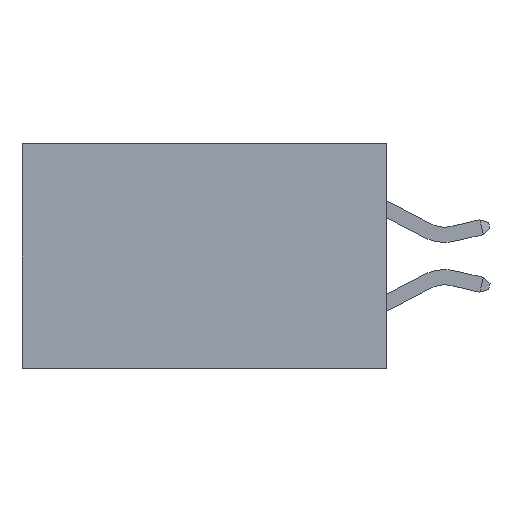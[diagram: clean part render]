
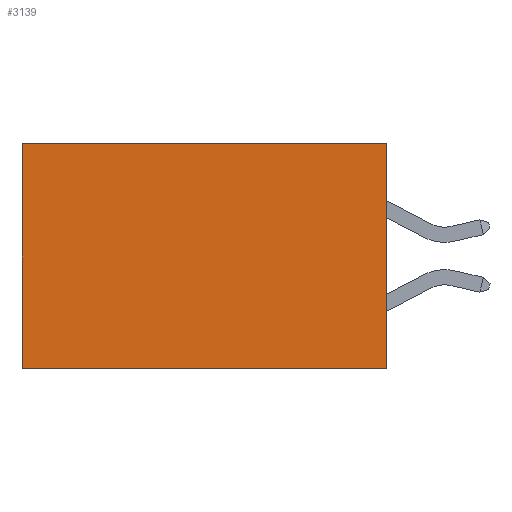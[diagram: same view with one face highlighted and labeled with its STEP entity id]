
A CAD part, left-side view. The second image highlights one B-rep face of the part: STEP entity #3139.
In plain terms, the highlighted planar face has unit normal (-1, 0, 0).
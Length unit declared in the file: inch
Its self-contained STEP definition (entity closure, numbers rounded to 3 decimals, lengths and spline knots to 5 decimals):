
#205 = VECTOR ( 'NONE', #7128, 39.37008 ) ;
#411 = LINE ( 'NONE', #13091, #9566 ) ;
#549 = VERTEX_POINT ( 'NONE', #5265 ) ;
#751 = LINE ( 'NONE', #3924, #11899 ) ;
#807 = DIRECTION ( 'NONE',  ( 0., 0., -1. ) ) ;
#1482 = VERTEX_POINT ( 'NONE', #13178 ) ;
#1638 = DIRECTION ( 'NONE',  ( 0., 1., 0. ) ) ;
#1924 = DIRECTION ( 'NONE',  ( 0., 0., -1. ) ) ;
#2231 = DIRECTION ( 'NONE',  ( 1., 0., 0. ) ) ;
#2800 = ORIENTED_EDGE ( 'NONE', *, *, #12934, .T. ) ;
#3053 = CARTESIAN_POINT ( 'NONE',  ( 0.2615, 0., 0. ) ) ;
#3139 = ADVANCED_FACE ( 'NONE', ( #7653 ), #4467, .F. ) ;
#3297 = LINE ( 'NONE', #7434, #205 ) ;
#3339 = LINE ( 'NONE', #9926, #11431 ) ;
#3765 = CARTESIAN_POINT ( 'NONE',  ( 0.2615, 0., -0.37 ) ) ;
#3924 = CARTESIAN_POINT ( 'NONE',  ( 0.2615, 0., 0. ) ) ;
#4284 = EDGE_LOOP ( 'NONE', ( #5016, #10656, #5382, #2800 ) ) ;
#4467 = PLANE ( 'NONE',  #4517 ) ;
#4517 = AXIS2_PLACEMENT_3D ( 'NONE', #3765, #2231, #1924 ) ;
#5016 = ORIENTED_EDGE ( 'NONE', *, *, #12968, .T. ) ;
#5265 = CARTESIAN_POINT ( 'NONE',  ( 0.2615, 0.6, -0.37 ) ) ;
#5382 = ORIENTED_EDGE ( 'NONE', *, *, #6686, .F. ) ;
#6686 = EDGE_CURVE ( 'NONE', #11420, #12044, #3297, .T. ) ;
#7128 = DIRECTION ( 'NONE',  ( 0., 0., -1. ) ) ;
#7434 = CARTESIAN_POINT ( 'NONE',  ( 0.2615, 0., -0.37 ) ) ;
#7653 = FACE_OUTER_BOUND ( 'NONE', #4284, .T. ) ;
#9566 = VECTOR ( 'NONE', #807, 39.37008 ) ;
#9777 = DIRECTION ( 'NONE',  ( 0., 1., 0. ) ) ;
#9926 = CARTESIAN_POINT ( 'NONE',  ( 0.2615, 0., -0.37 ) ) ;
#10656 = ORIENTED_EDGE ( 'NONE', *, *, #13204, .F. ) ;
#11420 = VERTEX_POINT ( 'NONE', #3053 ) ;
#11431 = VECTOR ( 'NONE', #9777, 39.37008 ) ;
#11899 = VECTOR ( 'NONE', #1638, 39.37008 ) ;
#12044 = VERTEX_POINT ( 'NONE', #12380 ) ;
#12380 = CARTESIAN_POINT ( 'NONE',  ( 0.2615, 0., -0.37 ) ) ;
#12934 = EDGE_CURVE ( 'NONE', #11420, #1482, #751, .T. ) ;
#12968 = EDGE_CURVE ( 'NONE', #1482, #549, #411, .T. ) ;
#13091 = CARTESIAN_POINT ( 'NONE',  ( 0.2615, 0.6, -0.37 ) ) ;
#13178 = CARTESIAN_POINT ( 'NONE',  ( 0.2615, 0.6, 0. ) ) ;
#13204 = EDGE_CURVE ( 'NONE', #12044, #549, #3339, .T. ) ;
